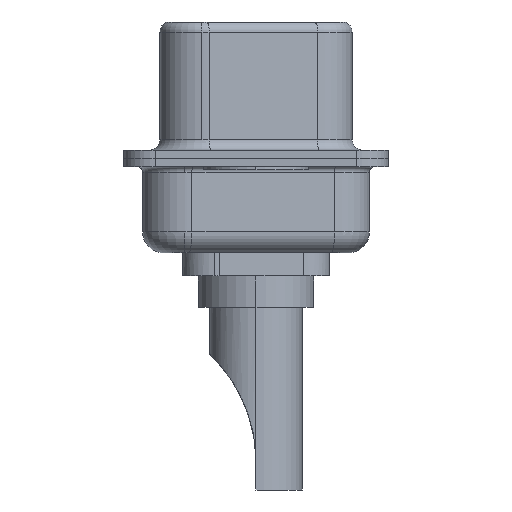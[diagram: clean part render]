
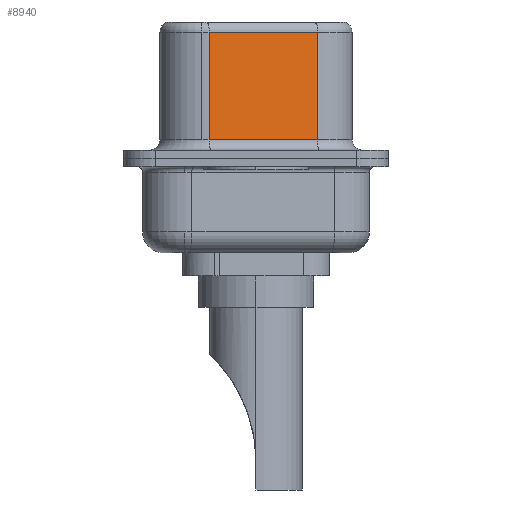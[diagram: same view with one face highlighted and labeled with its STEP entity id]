
A CAD part, left-side view. The second image highlights one B-rep face of the part: STEP entity #8940.
In plain terms, the highlighted planar face has unit normal (-0.985, -0.174, 0).
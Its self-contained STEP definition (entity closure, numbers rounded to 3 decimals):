
#84 = DIRECTION ( 'NONE',  ( -0.174, 0.985, 0. ) ) ;
#867 = AXIS2_PLACEMENT_3D ( 'NONE', #7231, #6040, #14453 ) ;
#1242 = CARTESIAN_POINT ( 'NONE',  ( 3.675, 2.233, 6.02 ) ) ;
#1606 = VECTOR ( 'NONE', #3275, 1000. ) ;
#1906 = ORIENTED_EDGE ( 'NONE', *, *, #5686, .T. ) ;
#2077 = VERTEX_POINT ( 'NONE', #1242 ) ;
#2385 = PLANE ( 'NONE',  #867 ) ;
#2412 = FACE_OUTER_BOUND ( 'NONE', #4925, .T. ) ;
#2705 = LINE ( 'NONE', #3771, #5932 ) ;
#3275 = DIRECTION ( 'NONE',  ( 0., 0., -1. ) ) ;
#3771 = CARTESIAN_POINT ( 'NONE',  ( 4.585, -2.927, 6.02 ) ) ;
#4477 = CARTESIAN_POINT ( 'NONE',  ( 3.675, 2.233, 6.52 ) ) ;
#4840 = VERTEX_POINT ( 'NONE', #15618 ) ;
#4925 = EDGE_LOOP ( 'NONE', ( #9823, #1906, #15124, #10777 ) ) ;
#5056 = EDGE_CURVE ( 'NONE', #4840, #5084, #6546, .T. ) ;
#5084 = VERTEX_POINT ( 'NONE', #14129 ) ;
#5686 = EDGE_CURVE ( 'NONE', #4840, #2077, #2705, .T. ) ;
#5932 = VECTOR ( 'NONE', #84, 1000. ) ;
#6040 = DIRECTION ( 'NONE',  ( 0.985, 0.174, 0. ) ) ;
#6546 = LINE ( 'NONE', #8508, #9318 ) ;
#6649 = VECTOR ( 'NONE', #9298, 1000. ) ;
#7027 = LINE ( 'NONE', #15322, #6649 ) ;
#7231 = CARTESIAN_POINT ( 'NONE',  ( 4.585, -2.927, 6.52 ) ) ;
#7667 = CARTESIAN_POINT ( 'NONE',  ( 3.675, 2.233, 0.9 ) ) ;
#8508 = CARTESIAN_POINT ( 'NONE',  ( 4.585, -2.927, 6.52 ) ) ;
#8618 = DIRECTION ( 'NONE',  ( 0., 0., -1. ) ) ;
#8940 = ADVANCED_FACE ( 'NONE', ( #2412 ), #2385, .F. ) ;
#9298 = DIRECTION ( 'NONE',  ( 0.174, -0.985, 0. ) ) ;
#9318 = VECTOR ( 'NONE', #8618, 1000. ) ;
#9823 = ORIENTED_EDGE ( 'NONE', *, *, #5056, .F. ) ;
#10777 = ORIENTED_EDGE ( 'NONE', *, *, #11497, .T. ) ;
#11207 = VERTEX_POINT ( 'NONE', #7667 ) ;
#11229 = LINE ( 'NONE', #4477, #1606 ) ;
#11497 = EDGE_CURVE ( 'NONE', #11207, #5084, #7027, .T. ) ;
#14129 = CARTESIAN_POINT ( 'NONE',  ( 4.585, -2.927, 0.9 ) ) ;
#14453 = DIRECTION ( 'NONE',  ( -0.174, 0.985, 0. ) ) ;
#15075 = EDGE_CURVE ( 'NONE', #2077, #11207, #11229, .T. ) ;
#15124 = ORIENTED_EDGE ( 'NONE', *, *, #15075, .T. ) ;
#15322 = CARTESIAN_POINT ( 'NONE',  ( 4.585, -2.927, 0.9 ) ) ;
#15618 = CARTESIAN_POINT ( 'NONE',  ( 4.585, -2.927, 6.02 ) ) ;
